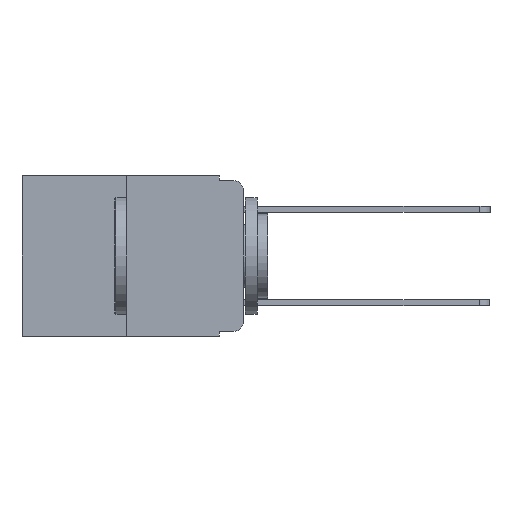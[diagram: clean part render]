
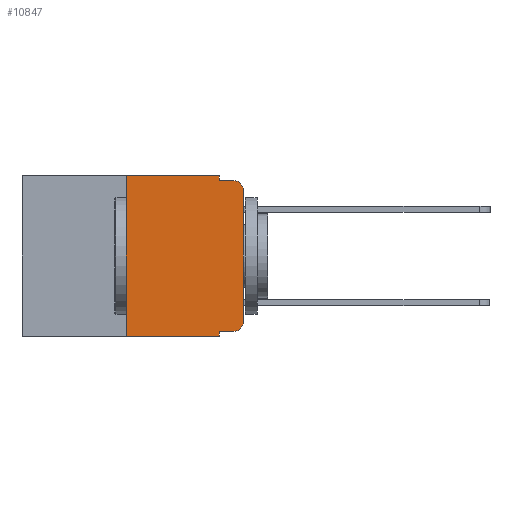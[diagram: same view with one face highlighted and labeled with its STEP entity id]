
A CAD part, left-side view. The second image highlights one B-rep face of the part: STEP entity #10847.
In plain terms, the highlighted planar face has unit normal (-1, 0, 0).
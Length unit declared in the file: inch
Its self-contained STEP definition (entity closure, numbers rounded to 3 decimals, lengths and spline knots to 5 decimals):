
#351 = DIRECTION ( 'NONE',  ( 0., -1., 0. ) ) ;
#740 = EDGE_CURVE ( 'NONE', #15139, #4687, #18613, .T. ) ;
#848 = CARTESIAN_POINT ( 'NONE',  ( 0., 0.051, -0.01 ) ) ;
#1061 = CARTESIAN_POINT ( 'NONE',  ( 0., 0.02, -0.01 ) ) ;
#1416 = CARTESIAN_POINT ( 'NONE',  ( 0., 0.051, -0.01 ) ) ;
#1623 = CARTESIAN_POINT ( 'NONE',  ( 0., 0.02, -0.333 ) ) ;
#1780 = CARTESIAN_POINT ( 'NONE',  ( 0., 0.051, 0. ) ) ;
#1987 = LINE ( 'NONE', #11258, #5952 ) ;
#2005 = EDGE_CURVE ( 'NONE', #4687, #2327, #8938, .T. ) ;
#2267 = DIRECTION ( 'NONE',  ( 0., -1., 0. ) ) ;
#2327 = VERTEX_POINT ( 'NONE', #1061 ) ;
#2348 = CIRCLE ( 'NONE', #13738, 0.02 ) ;
#2569 = ORIENTED_EDGE ( 'NONE', *, *, #7665, .F. ) ;
#2633 = CARTESIAN_POINT ( 'NONE',  ( 0., 0.051, -0.333 ) ) ;
#2669 = CARTESIAN_POINT ( 'NONE',  ( 0., 0.473, -0.343 ) ) ;
#2969 = VECTOR ( 'NONE', #5423, 39.37008 ) ;
#3405 = VECTOR ( 'NONE', #351, 39.37008 ) ;
#3714 = CARTESIAN_POINT ( 'NONE',  ( 0., 0.02, -0.03 ) ) ;
#3976 = ORIENTED_EDGE ( 'NONE', *, *, #17528, .F. ) ;
#4110 = CARTESIAN_POINT ( 'NONE',  ( 0., 0.02, -0.313 ) ) ;
#4318 = VECTOR ( 'NONE', #2267, 39.37008 ) ;
#4394 = FACE_OUTER_BOUND ( 'NONE', #14531, .T. ) ;
#4678 = ORIENTED_EDGE ( 'NONE', *, *, #15179, .T. ) ;
#4687 = VERTEX_POINT ( 'NONE', #11975 ) ;
#5107 = ORIENTED_EDGE ( 'NONE', *, *, #17846, .F. ) ;
#5286 = EDGE_CURVE ( 'NONE', #7936, #15139, #2348, .T. ) ;
#5423 = DIRECTION ( 'NONE',  ( 0., 0., -1. ) ) ;
#5571 = DIRECTION ( 'NONE',  ( 0., 0., -1. ) ) ;
#5715 = DIRECTION ( 'NONE',  ( 0., -1., 0. ) ) ;
#5821 = ORIENTED_EDGE ( 'NONE', *, *, #5286, .T. ) ;
#5952 = VECTOR ( 'NONE', #6909, 39.37008 ) ;
#6232 = ORIENTED_EDGE ( 'NONE', *, *, #2005, .T. ) ;
#6832 = CARTESIAN_POINT ( 'NONE',  ( 0., 0.051, -0.343 ) ) ;
#6909 = DIRECTION ( 'NONE',  ( 0., 0., 1. ) ) ;
#7037 = CARTESIAN_POINT ( 'NONE',  ( 0., 0., -0.313 ) ) ;
#7155 = VECTOR ( 'NONE', #17042, 39.37008 ) ;
#7594 = ORIENTED_EDGE ( 'NONE', *, *, #15242, .F. ) ;
#7598 = VECTOR ( 'NONE', #5715, 39.37008 ) ;
#7665 = EDGE_CURVE ( 'NONE', #18222, #9227, #11154, .T. ) ;
#7672 = PLANE ( 'NONE',  #9127 ) ;
#7734 = CARTESIAN_POINT ( 'NONE',  ( 0., 0.473, 0. ) ) ;
#7852 = ORIENTED_EDGE ( 'NONE', *, *, #18711, .T. ) ;
#7936 = VERTEX_POINT ( 'NONE', #1623 ) ;
#8522 = CARTESIAN_POINT ( 'NONE',  ( 0., 0.25, -0.343 ) ) ;
#8739 = ORIENTED_EDGE ( 'NONE', *, *, #740, .T. ) ;
#8938 = CIRCLE ( 'NONE', #18631, 0.02 ) ;
#9127 = AXIS2_PLACEMENT_3D ( 'NONE', #7734, #17778, #9203 ) ;
#9203 = DIRECTION ( 'NONE',  ( 0., 0., -1. ) ) ;
#9227 = VERTEX_POINT ( 'NONE', #6832 ) ;
#9885 = CARTESIAN_POINT ( 'NONE',  ( 0., 0.051, 0. ) ) ;
#10538 = VECTOR ( 'NONE', #11640, 39.37008 ) ;
#10559 = DIRECTION ( 'NONE',  ( 0., 0., -1. ) ) ;
#10847 = ADVANCED_FACE ( 'NONE', ( #4394 ), #7672, .F. ) ;
#11132 = LINE ( 'NONE', #13487, #3405 ) ;
#11154 = LINE ( 'NONE', #12608, #2969 ) ;
#11258 = CARTESIAN_POINT ( 'NONE',  ( 0., 0.25, 0. ) ) ;
#11640 = DIRECTION ( 'NONE',  ( 0., -1., 0. ) ) ;
#11975 = CARTESIAN_POINT ( 'NONE',  ( 0., 0., -0.03 ) ) ;
#11992 = LINE ( 'NONE', #16727, #4318 ) ;
#12196 = CARTESIAN_POINT ( 'NONE',  ( 0., 0., 0. ) ) ;
#12608 = CARTESIAN_POINT ( 'NONE',  ( 0., 0.051, 0. ) ) ;
#13487 = CARTESIAN_POINT ( 'NONE',  ( 0., 0.473, 0. ) ) ;
#13738 = AXIS2_PLACEMENT_3D ( 'NONE', #4110, #14174, #5571 ) ;
#13891 = LINE ( 'NONE', #1416, #10538 ) ;
#13922 = DIRECTION ( 'NONE',  ( 0., 0., -1. ) ) ;
#14002 = DIRECTION ( 'NONE',  ( -1., 0., 0. ) ) ;
#14174 = DIRECTION ( 'NONE',  ( -1., 0., 0. ) ) ;
#14531 = EDGE_LOOP ( 'NONE', ( #8739, #6232, #7594, #5107, #17044, #3976, #4678, #2569, #7852, #5821 ) ) ;
#14878 = CARTESIAN_POINT ( 'NONE',  ( 0., 0.25, 0. ) ) ;
#14941 = LINE ( 'NONE', #1780, #18749 ) ;
#15139 = VERTEX_POINT ( 'NONE', #7037 ) ;
#15152 = VERTEX_POINT ( 'NONE', #8522 ) ;
#15179 = EDGE_CURVE ( 'NONE', #15152, #9227, #15241, .T. ) ;
#15241 = LINE ( 'NONE', #2669, #7598 ) ;
#15242 = EDGE_CURVE ( 'NONE', #16880, #2327, #13891, .T. ) ;
#16727 = CARTESIAN_POINT ( 'NONE',  ( 0., 0.051, -0.333 ) ) ;
#16880 = VERTEX_POINT ( 'NONE', #848 ) ;
#17042 = DIRECTION ( 'NONE',  ( 0., 0., 1. ) ) ;
#17044 = ORIENTED_EDGE ( 'NONE', *, *, #17885, .F. ) ;
#17528 = EDGE_CURVE ( 'NONE', #15152, #17870, #1987, .T. ) ;
#17778 = DIRECTION ( 'NONE',  ( 1., 0., 0. ) ) ;
#17846 = EDGE_CURVE ( 'NONE', #18165, #16880, #14941, .T. ) ;
#17870 = VERTEX_POINT ( 'NONE', #14878 ) ;
#17885 = EDGE_CURVE ( 'NONE', #17870, #18165, #11132, .T. ) ;
#18165 = VERTEX_POINT ( 'NONE', #9885 ) ;
#18222 = VERTEX_POINT ( 'NONE', #2633 ) ;
#18613 = LINE ( 'NONE', #12196, #7155 ) ;
#18631 = AXIS2_PLACEMENT_3D ( 'NONE', #3714, #14002, #13922 ) ;
#18711 = EDGE_CURVE ( 'NONE', #18222, #7936, #11992, .T. ) ;
#18749 = VECTOR ( 'NONE', #10559, 39.37008 ) ;
